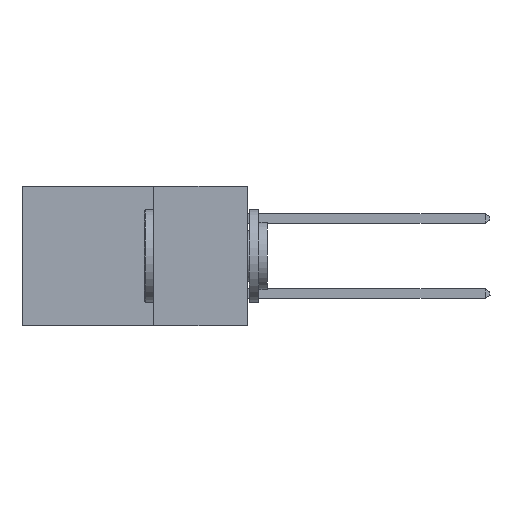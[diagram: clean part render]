
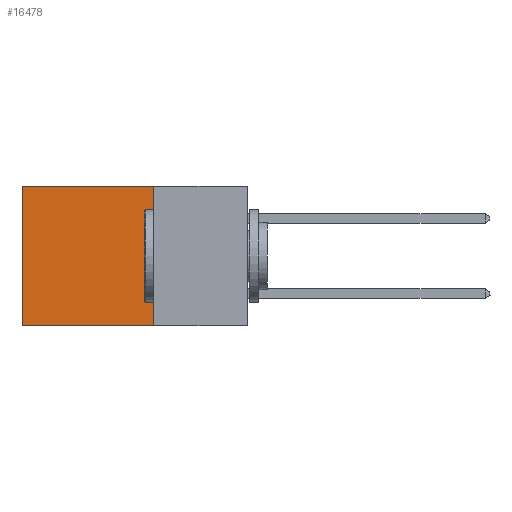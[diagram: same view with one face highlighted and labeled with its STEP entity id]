
A CAD part, left-side view. The second image highlights one B-rep face of the part: STEP entity #16478.
In plain terms, the highlighted planar face has unit normal (-1, 0, 0).
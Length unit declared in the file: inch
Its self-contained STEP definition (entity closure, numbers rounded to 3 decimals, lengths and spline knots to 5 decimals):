
#966 = VECTOR ( 'NONE', #7691, 39.37008 ) ;
#1479 = CARTESIAN_POINT ( 'NONE',  ( 0.298, 0.25, 0. ) ) ;
#1763 = EDGE_CURVE ( 'NONE', #4945, #19726, #10490, .T. ) ;
#2350 = DIRECTION ( 'NONE',  ( 1., 0., 0. ) ) ;
#2646 = VECTOR ( 'NONE', #19418, 39.37008 ) ;
#3087 = CARTESIAN_POINT ( 'NONE',  ( 0.298, 0.25, -0.37 ) ) ;
#3148 = CARTESIAN_POINT ( 'NONE',  ( 0.298, 0.6, 0. ) ) ;
#4113 = EDGE_LOOP ( 'NONE', ( #9380, #25552, #19962, #9713 ) ) ;
#4718 = DIRECTION ( 'NONE',  ( 0., 0., -1. ) ) ;
#4945 = VERTEX_POINT ( 'NONE', #5378 ) ;
#5378 = CARTESIAN_POINT ( 'NONE',  ( 0.298, 0.25, 0. ) ) ;
#6203 = DIRECTION ( 'NONE',  ( 0., 0., -1. ) ) ;
#7691 = DIRECTION ( 'NONE',  ( 0., 1., 0. ) ) ;
#9151 = LINE ( 'NONE', #21179, #966 ) ;
#9298 = LINE ( 'NONE', #10281, #14655 ) ;
#9380 = ORIENTED_EDGE ( 'NONE', *, *, #22278, .T. ) ;
#9713 = ORIENTED_EDGE ( 'NONE', *, *, #16120, .T. ) ;
#9777 = LINE ( 'NONE', #14866, #2646 ) ;
#10281 = CARTESIAN_POINT ( 'NONE',  ( 0.298, 0.6, 0. ) ) ;
#10490 = LINE ( 'NONE', #1479, #21841 ) ;
#11336 = CARTESIAN_POINT ( 'NONE',  ( 0.298, 0.25, 0. ) ) ;
#12377 = FACE_OUTER_BOUND ( 'NONE', #4113, .T. ) ;
#14655 = VECTOR ( 'NONE', #14782, 39.37008 ) ;
#14782 = DIRECTION ( 'NONE',  ( 0., 0., -1. ) ) ;
#14866 = CARTESIAN_POINT ( 'NONE',  ( 0.298, 0.25, -0.37 ) ) ;
#16120 = EDGE_CURVE ( 'NONE', #4945, #22651, #9151, .T. ) ;
#16478 = ADVANCED_FACE ( 'NONE', ( #12377 ), #26547, .F. ) ;
#17438 = VERTEX_POINT ( 'NONE', #23773 ) ;
#17733 = EDGE_CURVE ( 'NONE', #19726, #17438, #9777, .T. ) ;
#19418 = DIRECTION ( 'NONE',  ( 0., 1., 0. ) ) ;
#19726 = VERTEX_POINT ( 'NONE', #3087 ) ;
#19962 = ORIENTED_EDGE ( 'NONE', *, *, #1763, .F. ) ;
#21179 = CARTESIAN_POINT ( 'NONE',  ( 0.298, 0.25, 0. ) ) ;
#21841 = VECTOR ( 'NONE', #6203, 39.37008 ) ;
#22278 = EDGE_CURVE ( 'NONE', #22651, #17438, #9298, .T. ) ;
#22651 = VERTEX_POINT ( 'NONE', #3148 ) ;
#23773 = CARTESIAN_POINT ( 'NONE',  ( 0.298, 0.6, -0.37 ) ) ;
#25552 = ORIENTED_EDGE ( 'NONE', *, *, #17733, .F. ) ;
#26547 = PLANE ( 'NONE',  #28141 ) ;
#28141 = AXIS2_PLACEMENT_3D ( 'NONE', #11336, #2350, #4718 ) ;
